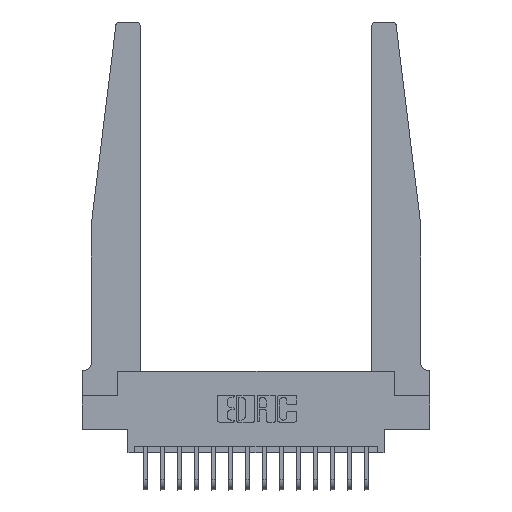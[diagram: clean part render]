
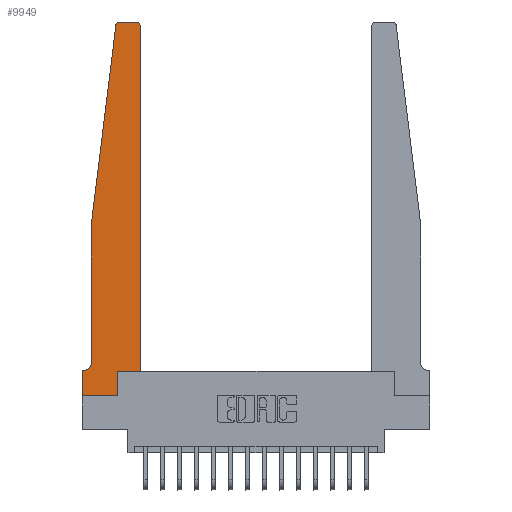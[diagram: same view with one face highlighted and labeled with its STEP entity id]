
A CAD part, top view. The second image highlights one B-rep face of the part: STEP entity #9949.
In plain terms, the highlighted planar face has unit normal (0, 0, 1).
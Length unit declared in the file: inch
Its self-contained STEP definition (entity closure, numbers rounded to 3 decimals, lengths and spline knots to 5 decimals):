
#15 = VERTEX_POINT ( 'NONE', #19683 ) ;
#378 = PLANE ( 'NONE',  #13714 ) ;
#698 = CARTESIAN_POINT ( 'NONE',  ( 0.425, 0.18, 0.37 ) ) ;
#720 = EDGE_CURVE ( 'NONE', #838, #7638, #10721, .T. ) ;
#838 = VERTEX_POINT ( 'NONE', #14040 ) ;
#1269 = ORIENTED_EDGE ( 'NONE', *, *, #12069, .T. ) ;
#1504 = LINE ( 'NONE', #18424, #15386 ) ;
#1791 = VECTOR ( 'NONE', #2703, 39.37008 ) ;
#1911 = DIRECTION ( 'NONE',  ( 0., 0., 1. ) ) ;
#2058 = CIRCLE ( 'NONE', #17278, 0.03 ) ;
#2213 = EDGE_CURVE ( 'NONE', #2533, #3289, #2469, .T. ) ;
#2459 = EDGE_CURVE ( 'NONE', #2538, #17134, #8616, .T. ) ;
#2469 = LINE ( 'NONE', #19583, #10024 ) ;
#2533 = VERTEX_POINT ( 'NONE', #14995 ) ;
#2538 = VERTEX_POINT ( 'NONE', #8740 ) ;
#2703 = DIRECTION ( 'NONE',  ( 0., -1., 0. ) ) ;
#3111 = DIRECTION ( 'NONE',  ( -0.122, -0.992, 0. ) ) ;
#3177 = LINE ( 'NONE', #17170, #18821 ) ;
#3289 = VERTEX_POINT ( 'NONE', #8524 ) ;
#3539 = CARTESIAN_POINT ( 'NONE',  ( 0., 0.1875, 0.37 ) ) ;
#3601 = CARTESIAN_POINT ( 'NONE',  ( 0.425, 2.72, 0.37 ) ) ;
#3762 = DIRECTION ( 'NONE',  ( 0., 0., 1. ) ) ;
#4296 = DIRECTION ( 'NONE',  ( -1., 0., 0. ) ) ;
#5046 = DIRECTION ( 'NONE',  ( 1., 0., 0. ) ) ;
#5135 = CARTESIAN_POINT ( 'NONE',  ( 0., 0.1875, 0.37 ) ) ;
#5889 = AXIS2_PLACEMENT_3D ( 'NONE', #19750, #11986, #7612 ) ;
#5928 = EDGE_CURVE ( 'NONE', #15, #7992, #12696, .T. ) ;
#6578 = DIRECTION ( 'NONE',  ( 1., 0., 0. ) ) ;
#6831 = ORIENTED_EDGE ( 'NONE', *, *, #13182, .T. ) ;
#6902 = VECTOR ( 'NONE', #5046, 39.37008 ) ;
#6917 = CARTESIAN_POINT ( 'NONE',  ( 0.065, 1.25, 0.37 ) ) ;
#7612 = DIRECTION ( 'NONE',  ( 1., 0., 0. ) ) ;
#7638 = VERTEX_POINT ( 'NONE', #3601 ) ;
#7956 = CARTESIAN_POINT ( 'NONE',  ( 0.065, 1.25, 0.37 ) ) ;
#7992 = VERTEX_POINT ( 'NONE', #18866 ) ;
#8141 = DIRECTION ( 'NONE',  ( -1., 0., 0. ) ) ;
#8278 = ORIENTED_EDGE ( 'NONE', *, *, #5928, .T. ) ;
#8433 = EDGE_CURVE ( 'NONE', #3289, #838, #19244, .T. ) ;
#8445 = LINE ( 'NONE', #6917, #11425 ) ;
#8524 = CARTESIAN_POINT ( 'NONE',  ( 0.2605, 0.18, 0.37 ) ) ;
#8616 = CIRCLE ( 'NONE', #16041, 0.05 ) ;
#8740 = CARTESIAN_POINT ( 'NONE',  ( 0.065, 0.2375, 0.37 ) ) ;
#8755 = CARTESIAN_POINT ( 'NONE',  ( 0.395, 2.75, 0.37 ) ) ;
#8871 = ORIENTED_EDGE ( 'NONE', *, *, #2213, .T. ) ;
#8954 = ORIENTED_EDGE ( 'NONE', *, *, #16670, .T. ) ;
#8996 = CARTESIAN_POINT ( 'NONE',  ( 0.425, 0.18, 0.37 ) ) ;
#9868 = VECTOR ( 'NONE', #17825, 39.37008 ) ;
#9949 = ADVANCED_FACE ( 'NONE', ( #18528 ), #378, .T. ) ;
#10024 = VECTOR ( 'NONE', #19480, 39.37008 ) ;
#10028 = ORIENTED_EDGE ( 'NONE', *, *, #12939, .T. ) ;
#10242 = LINE ( 'NONE', #13155, #1791 ) ;
#10721 = LINE ( 'NONE', #8996, #13168 ) ;
#11042 = LINE ( 'NONE', #13963, #16610 ) ;
#11425 = VECTOR ( 'NONE', #14716, 39.37008 ) ;
#11517 = ORIENTED_EDGE ( 'NONE', *, *, #2459, .T. ) ;
#11640 = ORIENTED_EDGE ( 'NONE', *, *, #8433, .T. ) ;
#11693 = VERTEX_POINT ( 'NONE', #12978 ) ;
#11986 = DIRECTION ( 'NONE',  ( 0., 0., 1. ) ) ;
#12069 = EDGE_CURVE ( 'NONE', #13158, #15, #1504, .T. ) ;
#12354 = ORIENTED_EDGE ( 'NONE', *, *, #15759, .T. ) ;
#12696 = CIRCLE ( 'NONE', #5889, 0.03 ) ;
#12939 = EDGE_CURVE ( 'NONE', #17134, #13820, #3177, .T. ) ;
#12978 = CARTESIAN_POINT ( 'NONE',  ( 0., 0., 0.37 ) ) ;
#13155 = CARTESIAN_POINT ( 'NONE',  ( 0., 0., 0.37 ) ) ;
#13158 = VERTEX_POINT ( 'NONE', #8755 ) ;
#13168 = VECTOR ( 'NONE', #20010, 39.37008 ) ;
#13182 = EDGE_CURVE ( 'NONE', #19831, #2538, #8445, .T. ) ;
#13714 = AXIS2_PLACEMENT_3D ( 'NONE', #3539, #1911, #6578 ) ;
#13820 = VERTEX_POINT ( 'NONE', #5135 ) ;
#13826 = CARTESIAN_POINT ( 'NONE',  ( 0.015, 0.2375, 0.37 ) ) ;
#13963 = CARTESIAN_POINT ( 'NONE',  ( 0.065, 1.25, 0.37 ) ) ;
#14040 = CARTESIAN_POINT ( 'NONE',  ( 0.425, 0.18, 0.37 ) ) ;
#14261 = CARTESIAN_POINT ( 'NONE',  ( 0., 0., 0.37 ) ) ;
#14715 = ORIENTED_EDGE ( 'NONE', *, *, #15593, .T. ) ;
#14716 = DIRECTION ( 'NONE',  ( 0., -1., 0. ) ) ;
#14995 = CARTESIAN_POINT ( 'NONE',  ( 0.2605, 0., 0.37 ) ) ;
#15386 = VECTOR ( 'NONE', #15489, 39.37008 ) ;
#15489 = DIRECTION ( 'NONE',  ( -1., 0., 0. ) ) ;
#15593 = EDGE_CURVE ( 'NONE', #7992, #19831, #11042, .T. ) ;
#15759 = EDGE_CURVE ( 'NONE', #11693, #2533, #16077, .T. ) ;
#16041 = AXIS2_PLACEMENT_3D ( 'NONE', #13826, #19991, #4296 ) ;
#16077 = LINE ( 'NONE', #14261, #6902 ) ;
#16133 = CARTESIAN_POINT ( 'NONE',  ( 0.395, 2.72, 0.37 ) ) ;
#16610 = VECTOR ( 'NONE', #3111, 39.37008 ) ;
#16629 = ORIENTED_EDGE ( 'NONE', *, *, #18248, .T. ) ;
#16670 = EDGE_CURVE ( 'NONE', #7638, #13158, #2058, .T. ) ;
#17134 = VERTEX_POINT ( 'NONE', #19803 ) ;
#17170 = CARTESIAN_POINT ( 'NONE',  ( 0.065, 0.1875, 0.37 ) ) ;
#17278 = AXIS2_PLACEMENT_3D ( 'NONE', #16133, #3762, #19448 ) ;
#17825 = DIRECTION ( 'NONE',  ( 1., 0., 0. ) ) ;
#18248 = EDGE_CURVE ( 'NONE', #13820, #11693, #10242, .T. ) ;
#18424 = CARTESIAN_POINT ( 'NONE',  ( 0.25, 2.75, 0.37 ) ) ;
#18528 = FACE_OUTER_BOUND ( 'NONE', #18603, .T. ) ;
#18603 = EDGE_LOOP ( 'NONE', ( #1269, #8278, #14715, #6831, #11517, #10028, #16629, #12354, #8871, #11640, #19783, #8954 ) ) ;
#18821 = VECTOR ( 'NONE', #8141, 39.37008 ) ;
#18866 = CARTESIAN_POINT ( 'NONE',  ( 0.24675, 2.72367, 0.37 ) ) ;
#19244 = LINE ( 'NONE', #698, #9868 ) ;
#19448 = DIRECTION ( 'NONE',  ( 1., 0., 0. ) ) ;
#19480 = DIRECTION ( 'NONE',  ( 0., 1., 0. ) ) ;
#19583 = CARTESIAN_POINT ( 'NONE',  ( 0.2605, 0.18, 0.37 ) ) ;
#19683 = CARTESIAN_POINT ( 'NONE',  ( 0.27653, 2.75, 0.37 ) ) ;
#19750 = CARTESIAN_POINT ( 'NONE',  ( 0.27653, 2.72, 0.37 ) ) ;
#19783 = ORIENTED_EDGE ( 'NONE', *, *, #720, .T. ) ;
#19803 = CARTESIAN_POINT ( 'NONE',  ( 0.015, 0.1875, 0.37 ) ) ;
#19831 = VERTEX_POINT ( 'NONE', #7956 ) ;
#19991 = DIRECTION ( 'NONE',  ( 0., 0., -1. ) ) ;
#20010 = DIRECTION ( 'NONE',  ( 0., 1., 0. ) ) ;
